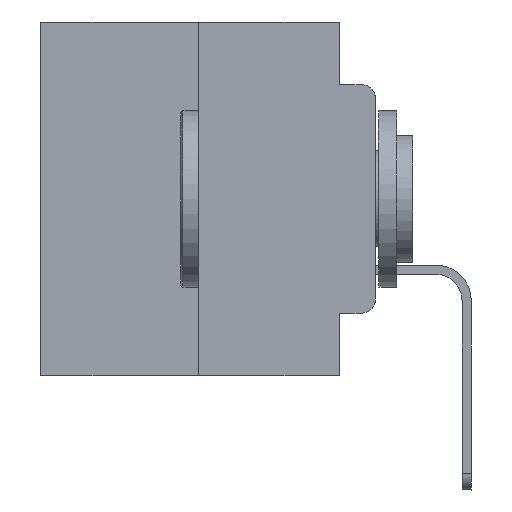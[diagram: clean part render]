
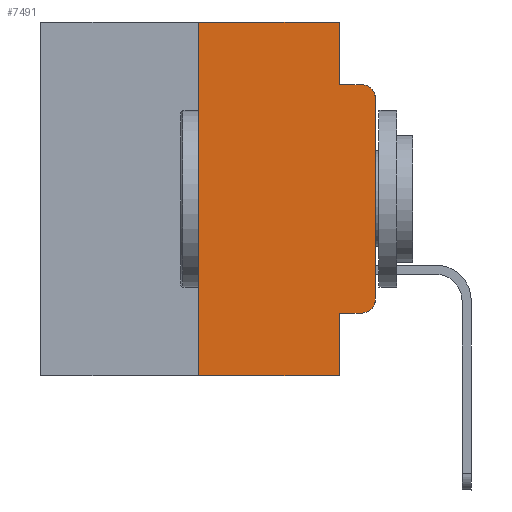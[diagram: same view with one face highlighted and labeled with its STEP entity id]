
A CAD part, left-side view. The second image highlights one B-rep face of the part: STEP entity #7491.
In plain terms, the highlighted planar face has unit normal (-1, 0, 0).
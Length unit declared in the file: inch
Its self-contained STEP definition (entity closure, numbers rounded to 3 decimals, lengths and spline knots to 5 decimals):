
#93 = VECTOR ( 'NONE', #25289, 39.37008 ) ;
#387 = ORIENTED_EDGE ( 'NONE', *, *, #16379, .T. ) ;
#626 = CIRCLE ( 'NONE', #11444, 0.02 ) ;
#1161 = VERTEX_POINT ( 'NONE', #8821 ) ;
#1323 = DIRECTION ( 'NONE',  ( 0., 0., -1. ) ) ;
#1718 = VERTEX_POINT ( 'NONE', #5684 ) ;
#2041 = DIRECTION ( 'NONE',  ( 0., 0., 1. ) ) ;
#2296 = CARTESIAN_POINT ( 'NONE',  ( 0., 0.25, 0. ) ) ;
#2600 = CARTESIAN_POINT ( 'NONE',  ( 0., 0.02, -0.4115 ) ) ;
#2609 = VERTEX_POINT ( 'NONE', #2600 ) ;
#2798 = CARTESIAN_POINT ( 'NONE',  ( 0., 0.051, 0. ) ) ;
#3052 = EDGE_CURVE ( 'NONE', #23774, #2609, #8479, .T. ) ;
#3110 = CARTESIAN_POINT ( 'NONE',  ( 0., 0.25, 0. ) ) ;
#3212 = EDGE_CURVE ( 'NONE', #17878, #11828, #19507, .T. ) ;
#3503 = DIRECTION ( 'NONE',  ( 0., 0., -1. ) ) ;
#3823 = LINE ( 'NONE', #10230, #12965 ) ;
#3952 = EDGE_CURVE ( 'NONE', #11329, #23314, #4198, .T. ) ;
#4047 = EDGE_CURVE ( 'NONE', #2609, #1718, #626, .T. ) ;
#4198 = LINE ( 'NONE', #3110, #21384 ) ;
#4505 = ORIENTED_EDGE ( 'NONE', *, *, #4677, .F. ) ;
#4677 = EDGE_CURVE ( 'NONE', #12125, #1161, #25266, .T. ) ;
#4683 = VERTEX_POINT ( 'NONE', #11029 ) ;
#5684 = CARTESIAN_POINT ( 'NONE',  ( 0., 0., -0.3915 ) ) ;
#5933 = LINE ( 'NONE', #8790, #93 ) ;
#6249 = ORIENTED_EDGE ( 'NONE', *, *, #3052, .T. ) ;
#6416 = CARTESIAN_POINT ( 'NONE',  ( 0., 0.473, -0.5 ) ) ;
#6739 = VECTOR ( 'NONE', #13311, 39.37008 ) ;
#7491 = ADVANCED_FACE ( 'NONE', ( #19338 ), #9534, .F. ) ;
#7694 = CARTESIAN_POINT ( 'NONE',  ( 0., 0.473, 0. ) ) ;
#8479 = LINE ( 'NONE', #11897, #15962 ) ;
#8583 = ORIENTED_EDGE ( 'NONE', *, *, #26222, .F. ) ;
#8746 = VECTOR ( 'NONE', #3503, 39.37008 ) ;
#8790 = CARTESIAN_POINT ( 'NONE',  ( 0., 0.473, 0. ) ) ;
#8821 = CARTESIAN_POINT ( 'NONE',  ( 0., 0.051, -0.0885 ) ) ;
#9534 = PLANE ( 'NONE',  #26436 ) ;
#9754 = ORIENTED_EDGE ( 'NONE', *, *, #21602, .F. ) ;
#10149 = DIRECTION ( 'NONE',  ( 0., -1., 0. ) ) ;
#10230 = CARTESIAN_POINT ( 'NONE',  ( 0., 0., 0. ) ) ;
#11029 = CARTESIAN_POINT ( 'NONE',  ( 0., 0.051, -0.5 ) ) ;
#11329 = VERTEX_POINT ( 'NONE', #21471 ) ;
#11444 = AXIS2_PLACEMENT_3D ( 'NONE', #21851, #22131, #17833 ) ;
#11462 = CARTESIAN_POINT ( 'NONE',  ( 0., 0.051, 0. ) ) ;
#11828 = VERTEX_POINT ( 'NONE', #12117 ) ;
#11897 = CARTESIAN_POINT ( 'NONE',  ( 0., 0.051, -0.4115 ) ) ;
#12117 = CARTESIAN_POINT ( 'NONE',  ( 0., 0.02, -0.0885 ) ) ;
#12125 = VERTEX_POINT ( 'NONE', #2798 ) ;
#12881 = LINE ( 'NONE', #6416, #16124 ) ;
#12894 = CARTESIAN_POINT ( 'NONE',  ( 0., 0.02, -0.1085 ) ) ;
#12965 = VECTOR ( 'NONE', #2041, 39.37008 ) ;
#13311 = DIRECTION ( 'NONE',  ( 0., 0., -1. ) ) ;
#13371 = DIRECTION ( 'NONE',  ( -1., 0., 0. ) ) ;
#13625 = ORIENTED_EDGE ( 'NONE', *, *, #14129, .F. ) ;
#14129 = EDGE_CURVE ( 'NONE', #23774, #4683, #23981, .T. ) ;
#14987 = DIRECTION ( 'NONE',  ( 0., -1., 0. ) ) ;
#15120 = EDGE_CURVE ( 'NONE', #1718, #17878, #3823, .T. ) ;
#15929 = ORIENTED_EDGE ( 'NONE', *, *, #15120, .T. ) ;
#15962 = VECTOR ( 'NONE', #10149, 39.37008 ) ;
#16124 = VECTOR ( 'NONE', #14987, 39.37008 ) ;
#16379 = EDGE_CURVE ( 'NONE', #11329, #4683, #12881, .T. ) ;
#17441 = ORIENTED_EDGE ( 'NONE', *, *, #3212, .T. ) ;
#17568 = DIRECTION ( 'NONE',  ( 0., 0., 1. ) ) ;
#17833 = DIRECTION ( 'NONE',  ( 0., 0., -1. ) ) ;
#17878 = VERTEX_POINT ( 'NONE', #19552 ) ;
#18628 = EDGE_LOOP ( 'NONE', ( #15929, #17441, #9754, #4505, #8583, #23257, #387, #13625, #6249, #21959 ) ) ;
#18864 = LINE ( 'NONE', #26242, #20453 ) ;
#19338 = FACE_OUTER_BOUND ( 'NONE', #18628, .T. ) ;
#19507 = CIRCLE ( 'NONE', #26502, 0.02 ) ;
#19552 = CARTESIAN_POINT ( 'NONE',  ( 0., 0., -0.1085 ) ) ;
#20043 = DIRECTION ( 'NONE',  ( 1., 0., 0. ) ) ;
#20244 = CARTESIAN_POINT ( 'NONE',  ( 0., 0.051, -0.4115 ) ) ;
#20453 = VECTOR ( 'NONE', #23876, 39.37008 ) ;
#21384 = VECTOR ( 'NONE', #17568, 39.37008 ) ;
#21471 = CARTESIAN_POINT ( 'NONE',  ( 0., 0.25, -0.5 ) ) ;
#21602 = EDGE_CURVE ( 'NONE', #1161, #11828, #18864, .T. ) ;
#21851 = CARTESIAN_POINT ( 'NONE',  ( 0., 0.02, -0.3915 ) ) ;
#21959 = ORIENTED_EDGE ( 'NONE', *, *, #4047, .T. ) ;
#22131 = DIRECTION ( 'NONE',  ( -1., 0., 0. ) ) ;
#22192 = DIRECTION ( 'NONE',  ( 0., 0., -1. ) ) ;
#23257 = ORIENTED_EDGE ( 'NONE', *, *, #3952, .F. ) ;
#23314 = VERTEX_POINT ( 'NONE', #2296 ) ;
#23774 = VERTEX_POINT ( 'NONE', #20244 ) ;
#23876 = DIRECTION ( 'NONE',  ( 0., -1., 0. ) ) ;
#23981 = LINE ( 'NONE', #11462, #8746 ) ;
#25266 = LINE ( 'NONE', #25687, #6739 ) ;
#25289 = DIRECTION ( 'NONE',  ( 0., -1., 0. ) ) ;
#25687 = CARTESIAN_POINT ( 'NONE',  ( 0., 0.051, 0. ) ) ;
#26222 = EDGE_CURVE ( 'NONE', #23314, #12125, #5933, .T. ) ;
#26242 = CARTESIAN_POINT ( 'NONE',  ( 0., 0.051, -0.0885 ) ) ;
#26436 = AXIS2_PLACEMENT_3D ( 'NONE', #7694, #20043, #22192 ) ;
#26502 = AXIS2_PLACEMENT_3D ( 'NONE', #12894, #13371, #1323 ) ;
